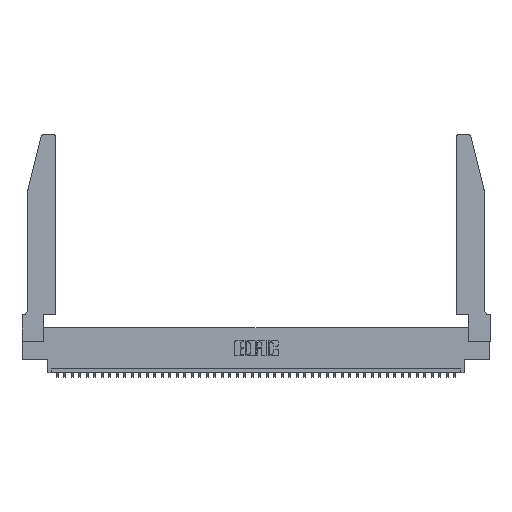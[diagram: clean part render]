
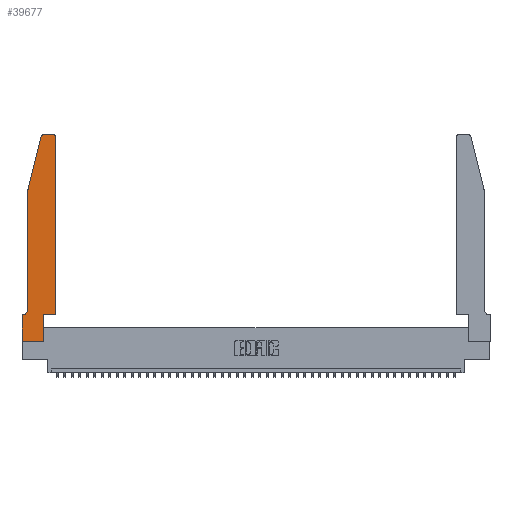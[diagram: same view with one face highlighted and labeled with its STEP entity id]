
A CAD part, top view. The second image highlights one B-rep face of the part: STEP entity #39677.
In plain terms, the highlighted planar face has unit normal (0, 0, 1).
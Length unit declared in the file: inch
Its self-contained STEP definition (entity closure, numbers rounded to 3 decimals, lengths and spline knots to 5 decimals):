
#852 = CARTESIAN_POINT ( 'NONE',  ( 0.284, 2.75, 0.37 ) ) ;
#934 = DIRECTION ( 'NONE',  ( 1., 0., 0. ) ) ;
#1536 = DIRECTION ( 'NONE',  ( -0.239, -0.971, 0. ) ) ;
#2064 = VECTOR ( 'NONE', #19049, 39.37008 ) ;
#2132 = VERTEX_POINT ( 'NONE', #24397 ) ;
#2453 = DIRECTION ( 'NONE',  ( 0., -1., 0. ) ) ;
#3847 = FACE_OUTER_BOUND ( 'NONE', #15553, .T. ) ;
#4151 = VECTOR ( 'NONE', #36762, 39.37008 ) ;
#4185 = LINE ( 'NONE', #9339, #39284 ) ;
#5126 = EDGE_CURVE ( 'NONE', #36408, #29139, #23756, .T. ) ;
#5474 = VECTOR ( 'NONE', #17929, 39.37008 ) ;
#5852 = CARTESIAN_POINT ( 'NONE',  ( 0., 0., 0.37 ) ) ;
#6935 = VECTOR ( 'NONE', #31704, 39.37008 ) ;
#7235 = ORIENTED_EDGE ( 'NONE', *, *, #42559, .T. ) ;
#7791 = CARTESIAN_POINT ( 'NONE',  ( 0.0055, 0.35, 0.37 ) ) ;
#7803 = DIRECTION ( 'NONE',  ( 0., 0., 1. ) ) ;
#7945 = LINE ( 'NONE', #24948, #6935 ) ;
#8377 = ORIENTED_EDGE ( 'NONE', *, *, #37187, .T. ) ;
#8669 = CARTESIAN_POINT ( 'NONE',  ( 0.25487, 2.72718, 0.37 ) ) ;
#9339 = CARTESIAN_POINT ( 'NONE',  ( 0.4505, 0.35, 0.37 ) ) ;
#9446 = CARTESIAN_POINT ( 'NONE',  ( 0.4205, 2.72, 0.37 ) ) ;
#9572 = VERTEX_POINT ( 'NONE', #31255 ) ;
#10443 = EDGE_CURVE ( 'NONE', #2132, #30298, #4185, .T. ) ;
#11684 = VERTEX_POINT ( 'NONE', #37271 ) ;
#11896 = EDGE_CURVE ( 'NONE', #12093, #12035, #38634, .T. ) ;
#12035 = VERTEX_POINT ( 'NONE', #30346 ) ;
#12093 = VERTEX_POINT ( 'NONE', #7791 ) ;
#12638 = ORIENTED_EDGE ( 'NONE', *, *, #5126, .T. ) ;
#13033 = AXIS2_PLACEMENT_3D ( 'NONE', #9446, #43579, #16270 ) ;
#14400 = ORIENTED_EDGE ( 'NONE', *, *, #33316, .T. ) ;
#15362 = LINE ( 'NONE', #15619, #2064 ) ;
#15553 = EDGE_LOOP ( 'NONE', ( #30889, #12638, #8377, #19224, #7235, #17696, #21744, #14400, #43891, #41550, #31538, #28183 ) ) ;
#15619 = CARTESIAN_POINT ( 'NONE',  ( 0.0755, 2., 0.37 ) ) ;
#15860 = LINE ( 'NONE', #5852, #4151 ) ;
#16075 = VECTOR ( 'NONE', #1536, 39.37008 ) ;
#16270 = DIRECTION ( 'NONE',  ( 1., 0., 0. ) ) ;
#16300 = EDGE_CURVE ( 'NONE', #30298, #11684, #17701, .T. ) ;
#17537 = DIRECTION ( 'NONE',  ( 1., 0., 0. ) ) ;
#17696 = ORIENTED_EDGE ( 'NONE', *, *, #11896, .T. ) ;
#17701 = LINE ( 'NONE', #24660, #5474 ) ;
#17924 = CARTESIAN_POINT ( 'NONE',  ( 0.2865, 0., 0.37 ) ) ;
#17929 = DIRECTION ( 'NONE',  ( 0., 1., 0. ) ) ;
#18184 = LINE ( 'NONE', #35139, #16075 ) ;
#18191 = EDGE_CURVE ( 'NONE', #42062, #36408, #7945, .T. ) ;
#18442 = VERTEX_POINT ( 'NONE', #33410 ) ;
#18537 = EDGE_CURVE ( 'NONE', #9572, #18442, #15362, .T. ) ;
#19049 = DIRECTION ( 'NONE',  ( 0., -1., 0. ) ) ;
#19224 = ORIENTED_EDGE ( 'NONE', *, *, #18537, .T. ) ;
#19593 = DIRECTION ( 'NONE',  ( -1., 0., 0. ) ) ;
#19999 = CARTESIAN_POINT ( 'NONE',  ( 0.0755, 0.35, 0.37 ) ) ;
#20124 = VERTEX_POINT ( 'NONE', #27758 ) ;
#21295 = AXIS2_PLACEMENT_3D ( 'NONE', #31424, #42821, #17537 ) ;
#21744 = ORIENTED_EDGE ( 'NONE', *, *, #31860, .T. ) ;
#22251 = CARTESIAN_POINT ( 'NONE',  ( 0., 0., 0.37 ) ) ;
#22446 = CARTESIAN_POINT ( 'NONE',  ( 0.4205, 2.75, 0.37 ) ) ;
#22781 = CIRCLE ( 'NONE', #40455, 0.07 ) ;
#22890 = DIRECTION ( 'NONE',  ( 1., 0., 0. ) ) ;
#23756 = CIRCLE ( 'NONE', #21295, 0.03 ) ;
#24397 = CARTESIAN_POINT ( 'NONE',  ( 0.2865, 0.35, 0.37 ) ) ;
#24537 = CIRCLE ( 'NONE', #13033, 0.03 ) ;
#24660 = CARTESIAN_POINT ( 'NONE',  ( 0.4505, 0.35, 0.37 ) ) ;
#24948 = CARTESIAN_POINT ( 'NONE',  ( 0.2605, 2.75, 0.37 ) ) ;
#25617 = VECTOR ( 'NONE', #2453, 39.37008 ) ;
#26893 = LINE ( 'NONE', #43957, #36368 ) ;
#27101 = DIRECTION ( 'NONE',  ( 0., 1., 0. ) ) ;
#27758 = CARTESIAN_POINT ( 'NONE',  ( 0., 0., 0.37 ) ) ;
#28043 = EDGE_CURVE ( 'NONE', #30021, #2132, #26893, .T. ) ;
#28183 = ORIENTED_EDGE ( 'NONE', *, *, #31974, .T. ) ;
#28301 = PLANE ( 'NONE',  #34134 ) ;
#29139 = VERTEX_POINT ( 'NONE', #8669 ) ;
#30021 = VERTEX_POINT ( 'NONE', #17924 ) ;
#30298 = VERTEX_POINT ( 'NONE', #40049 ) ;
#30346 = CARTESIAN_POINT ( 'NONE',  ( 0., 0.35, 0.37 ) ) ;
#30889 = ORIENTED_EDGE ( 'NONE', *, *, #18191, .T. ) ;
#31255 = CARTESIAN_POINT ( 'NONE',  ( 0.0755, 2., 0.37 ) ) ;
#31424 = CARTESIAN_POINT ( 'NONE',  ( 0.284, 2.72, 0.37 ) ) ;
#31538 = ORIENTED_EDGE ( 'NONE', *, *, #16300, .T. ) ;
#31704 = DIRECTION ( 'NONE',  ( -1., 0., 0. ) ) ;
#31860 = EDGE_CURVE ( 'NONE', #12035, #20124, #35658, .T. ) ;
#31974 = EDGE_CURVE ( 'NONE', #11684, #42062, #24537, .T. ) ;
#33074 = DIRECTION ( 'NONE',  ( 0., 0., -1. ) ) ;
#33316 = EDGE_CURVE ( 'NONE', #20124, #30021, #15860, .T. ) ;
#33410 = CARTESIAN_POINT ( 'NONE',  ( 0.0755, 0.42, 0.37 ) ) ;
#34134 = AXIS2_PLACEMENT_3D ( 'NONE', #41625, #7803, #934 ) ;
#35139 = CARTESIAN_POINT ( 'NONE',  ( 0.0755, 2., 0.37 ) ) ;
#35441 = VECTOR ( 'NONE', #37045, 39.37008 ) ;
#35658 = LINE ( 'NONE', #22251, #25617 ) ;
#36368 = VECTOR ( 'NONE', #27101, 39.37008 ) ;
#36408 = VERTEX_POINT ( 'NONE', #852 ) ;
#36762 = DIRECTION ( 'NONE',  ( 1., 0., 0. ) ) ;
#37045 = DIRECTION ( 'NONE',  ( -1., 0., 0. ) ) ;
#37187 = EDGE_CURVE ( 'NONE', #29139, #9572, #18184, .T. ) ;
#37271 = CARTESIAN_POINT ( 'NONE',  ( 0.4505, 2.72, 0.37 ) ) ;
#38634 = LINE ( 'NONE', #19999, #35441 ) ;
#39284 = VECTOR ( 'NONE', #22890, 39.37008 ) ;
#39677 = ADVANCED_FACE ( 'NONE', ( #3847 ), #28301, .T. ) ;
#39919 = CARTESIAN_POINT ( 'NONE',  ( 0.0055, 0.42, 0.37 ) ) ;
#40049 = CARTESIAN_POINT ( 'NONE',  ( 0.4505, 0.35, 0.37 ) ) ;
#40455 = AXIS2_PLACEMENT_3D ( 'NONE', #39919, #33074, #19593 ) ;
#41550 = ORIENTED_EDGE ( 'NONE', *, *, #10443, .T. ) ;
#41625 = CARTESIAN_POINT ( 'NONE',  ( 0., 0.35, 0.37 ) ) ;
#42062 = VERTEX_POINT ( 'NONE', #22446 ) ;
#42559 = EDGE_CURVE ( 'NONE', #18442, #12093, #22781, .T. ) ;
#42821 = DIRECTION ( 'NONE',  ( 0., 0., 1. ) ) ;
#43579 = DIRECTION ( 'NONE',  ( 0., 0., 1. ) ) ;
#43891 = ORIENTED_EDGE ( 'NONE', *, *, #28043, .T. ) ;
#43957 = CARTESIAN_POINT ( 'NONE',  ( 0.2865, 0.35, 0.37 ) ) ;
